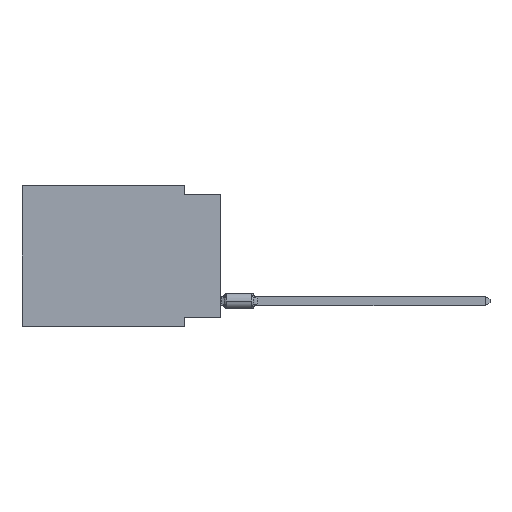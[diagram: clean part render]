
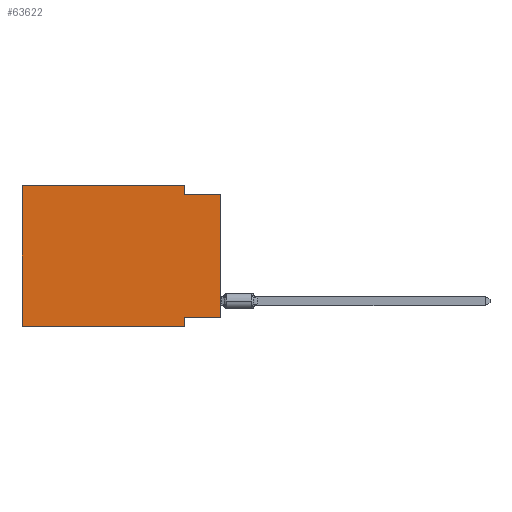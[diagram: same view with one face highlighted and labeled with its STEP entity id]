
A CAD part, left-side view. The second image highlights one B-rep face of the part: STEP entity #63622.
In plain terms, the highlighted planar face has unit normal (-1, 0, 0).
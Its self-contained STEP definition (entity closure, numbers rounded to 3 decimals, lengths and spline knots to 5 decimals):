
#1837 = VERTEX_POINT ( 'NONE', #56603 ) ;
#2078 = VECTOR ( 'NONE', #54040, 39.37008 ) ;
#2141 = LINE ( 'NONE', #24322, #60826 ) ;
#5561 = EDGE_CURVE ( 'NONE', #14350, #39160, #29230, .T. ) ;
#7489 = CARTESIAN_POINT ( 'NONE',  ( 0., 0.55, 0. ) ) ;
#8176 = VECTOR ( 'NONE', #13611, 39.37008 ) ;
#8793 = VECTOR ( 'NONE', #44299, 39.37008 ) ;
#8910 = CARTESIAN_POINT ( 'NONE',  ( 0., 0.55, 0. ) ) ;
#9172 = FACE_OUTER_BOUND ( 'NONE', #47164, .T. ) ;
#10647 = VERTEX_POINT ( 'NONE', #28903 ) ;
#11138 = CARTESIAN_POINT ( 'NONE',  ( 0., 0.1, -0.365 ) ) ;
#13135 = CARTESIAN_POINT ( 'NONE',  ( 0., 0., -0.025 ) ) ;
#13292 = LINE ( 'NONE', #7489, #8176 ) ;
#13611 = DIRECTION ( 'NONE',  ( 0., -1., 0. ) ) ;
#14290 = ORIENTED_EDGE ( 'NONE', *, *, #45234, .F. ) ;
#14333 = EDGE_CURVE ( 'NONE', #1837, #45866, #22592, .T. ) ;
#14350 = VERTEX_POINT ( 'NONE', #59179 ) ;
#14384 = LINE ( 'NONE', #8910, #29967 ) ;
#15644 = DIRECTION ( 'NONE',  ( 0., 0., -1. ) ) ;
#17232 = DIRECTION ( 'NONE',  ( 0., 0., 1. ) ) ;
#17802 = CARTESIAN_POINT ( 'NONE',  ( 0., 0., -0.365 ) ) ;
#17950 = CARTESIAN_POINT ( 'NONE',  ( 0., 0., -0.025 ) ) ;
#19787 = PLANE ( 'NONE',  #66960 ) ;
#21121 = CARTESIAN_POINT ( 'NONE',  ( 0., 0.55, 0. ) ) ;
#22592 = LINE ( 'NONE', #17802, #2078 ) ;
#23434 = CARTESIAN_POINT ( 'NONE',  ( 0., 0.1, 0. ) ) ;
#23702 = CARTESIAN_POINT ( 'NONE',  ( 0., 0., 0. ) ) ;
#23736 = CARTESIAN_POINT ( 'NONE',  ( 0., 0.1, -0.025 ) ) ;
#24322 = CARTESIAN_POINT ( 'NONE',  ( 0., 0.1, -0.39 ) ) ;
#26072 = EDGE_CURVE ( 'NONE', #39160, #53578, #44605, .T. ) ;
#26099 = EDGE_CURVE ( 'NONE', #49449, #39464, #28554, .T. ) ;
#26294 = ORIENTED_EDGE ( 'NONE', *, *, #14333, .F. ) ;
#28554 = LINE ( 'NONE', #34002, #29288 ) ;
#28903 = CARTESIAN_POINT ( 'NONE',  ( 0., 0.55, 0. ) ) ;
#29230 = LINE ( 'NONE', #23434, #8793 ) ;
#29288 = VECTOR ( 'NONE', #54873, 39.37008 ) ;
#29967 = VECTOR ( 'NONE', #61222, 39.37008 ) ;
#30010 = DIRECTION ( 'NONE',  ( 1., 0., 0. ) ) ;
#30350 = ORIENTED_EDGE ( 'NONE', *, *, #51254, .F. ) ;
#34002 = CARTESIAN_POINT ( 'NONE',  ( 0., 0.55, -0.39 ) ) ;
#35942 = EDGE_CURVE ( 'NONE', #10647, #14350, #13292, .T. ) ;
#36033 = VECTOR ( 'NONE', #17232, 39.37008 ) ;
#39160 = VERTEX_POINT ( 'NONE', #23736 ) ;
#39464 = VERTEX_POINT ( 'NONE', #57852 ) ;
#44299 = DIRECTION ( 'NONE',  ( 0., 0., -1. ) ) ;
#44605 = LINE ( 'NONE', #17950, #58789 ) ;
#45234 = EDGE_CURVE ( 'NONE', #45866, #39464, #2141, .T. ) ;
#45866 = VERTEX_POINT ( 'NONE', #11138 ) ;
#47164 = EDGE_LOOP ( 'NONE', ( #50624, #57005, #53961, #53938, #30350, #56077, #14290, #26294 ) ) ;
#48756 = EDGE_CURVE ( 'NONE', #1837, #53578, #64063, .T. ) ;
#49449 = VERTEX_POINT ( 'NONE', #53250 ) ;
#50624 = ORIENTED_EDGE ( 'NONE', *, *, #48756, .T. ) ;
#51254 = EDGE_CURVE ( 'NONE', #49449, #10647, #14384, .T. ) ;
#53250 = CARTESIAN_POINT ( 'NONE',  ( 0., 0.55, -0.39 ) ) ;
#53578 = VERTEX_POINT ( 'NONE', #13135 ) ;
#53938 = ORIENTED_EDGE ( 'NONE', *, *, #35942, .F. ) ;
#53961 = ORIENTED_EDGE ( 'NONE', *, *, #5561, .F. ) ;
#54040 = DIRECTION ( 'NONE',  ( 0., 1., 0. ) ) ;
#54771 = DIRECTION ( 'NONE',  ( 0., 0., -1. ) ) ;
#54873 = DIRECTION ( 'NONE',  ( 0., -1., 0. ) ) ;
#56077 = ORIENTED_EDGE ( 'NONE', *, *, #26099, .T. ) ;
#56603 = CARTESIAN_POINT ( 'NONE',  ( 0., 0., -0.365 ) ) ;
#57005 = ORIENTED_EDGE ( 'NONE', *, *, #26072, .F. ) ;
#57852 = CARTESIAN_POINT ( 'NONE',  ( 0., 0.1, -0.39 ) ) ;
#58789 = VECTOR ( 'NONE', #60317, 39.37008 ) ;
#59179 = CARTESIAN_POINT ( 'NONE',  ( 0., 0.1, 0. ) ) ;
#60317 = DIRECTION ( 'NONE',  ( 0., -1., 0. ) ) ;
#60826 = VECTOR ( 'NONE', #54771, 39.37008 ) ;
#61222 = DIRECTION ( 'NONE',  ( 0., 0., 1. ) ) ;
#63622 = ADVANCED_FACE ( 'NONE', ( #9172 ), #19787, .F. ) ;
#64063 = LINE ( 'NONE', #23702, #36033 ) ;
#66960 = AXIS2_PLACEMENT_3D ( 'NONE', #21121, #30010, #15644 ) ;
